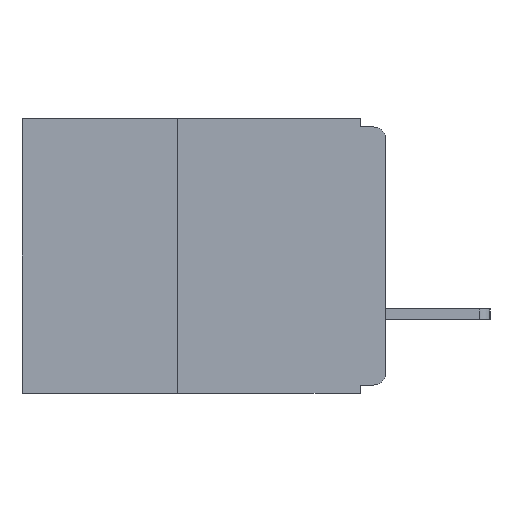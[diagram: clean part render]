
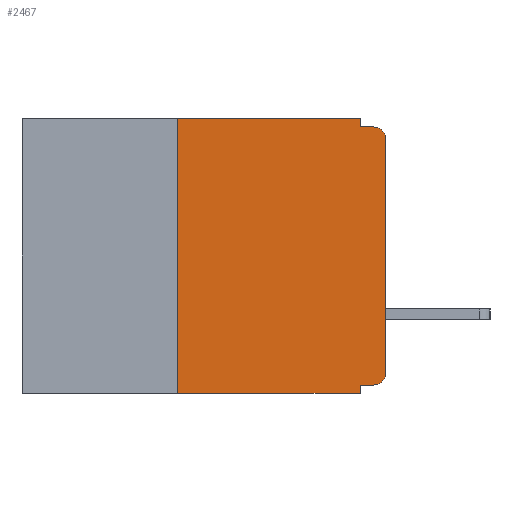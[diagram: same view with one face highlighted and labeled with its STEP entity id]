
A CAD part, left-side view. The second image highlights one B-rep face of the part: STEP entity #2467.
In plain terms, the highlighted planar face has unit normal (-1, 0, 0).
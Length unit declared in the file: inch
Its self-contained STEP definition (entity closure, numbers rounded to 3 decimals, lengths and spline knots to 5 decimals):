
#266 = DIRECTION ( 'NONE',  ( 0., 0., 1. ) ) ;
#405 = DIRECTION ( 'NONE',  ( 0., 0., -1. ) ) ;
#1133 = DIRECTION ( 'NONE',  ( -1., 0., 0. ) ) ;
#1836 = EDGE_CURVE ( 'NONE', #6928, #7403, #9628, .T. ) ;
#2467 = ADVANCED_FACE ( 'NONE', ( #5441 ), #2619, .F. ) ;
#2619 = PLANE ( 'NONE',  #10414 ) ;
#2712 = EDGE_CURVE ( 'NONE', #7403, #15019, #13500, .T. ) ;
#2730 = VECTOR ( 'NONE', #266, 39.37008 ) ;
#2902 = DIRECTION ( 'NONE',  ( 0., -1., 0. ) ) ;
#2996 = CARTESIAN_POINT ( 'NONE',  ( 0., 0.031, -0.01 ) ) ;
#3098 = EDGE_CURVE ( 'NONE', #8021, #14418, #10614, .T. ) ;
#3619 = ORIENTED_EDGE ( 'NONE', *, *, #6432, .F. ) ;
#3790 = DIRECTION ( 'NONE',  ( 0., -1., 0. ) ) ;
#4138 = CARTESIAN_POINT ( 'NONE',  ( 0., 0.015, -0.01 ) ) ;
#4578 = CARTESIAN_POINT ( 'NONE',  ( 0., 0., -0.01 ) ) ;
#4622 = VERTEX_POINT ( 'NONE', #8801 ) ;
#5047 = CARTESIAN_POINT ( 'NONE',  ( 0., 0., -0.305 ) ) ;
#5087 = VERTEX_POINT ( 'NONE', #5047 ) ;
#5209 = VECTOR ( 'NONE', #11795, 39.37008 ) ;
#5441 = FACE_OUTER_BOUND ( 'NONE', #16804, .T. ) ;
#5730 = AXIS2_PLACEMENT_3D ( 'NONE', #20215, #10373, #405 ) ;
#5821 = DIRECTION ( 'NONE',  ( 0., 0., -1. ) ) ;
#5935 = CARTESIAN_POINT ( 'NONE',  ( 0., 0., -0.32 ) ) ;
#6432 = EDGE_CURVE ( 'NONE', #18299, #6928, #12663, .T. ) ;
#6604 = ORIENTED_EDGE ( 'NONE', *, *, #2712, .F. ) ;
#6928 = VERTEX_POINT ( 'NONE', #10141 ) ;
#7403 = VERTEX_POINT ( 'NONE', #19286 ) ;
#7618 = DIRECTION ( 'NONE',  ( 0., 1., 0. ) ) ;
#8021 = VERTEX_POINT ( 'NONE', #16080 ) ;
#8182 = LINE ( 'NONE', #4578, #20773 ) ;
#8572 = CARTESIAN_POINT ( 'NONE',  ( 0., 0.25, -0.33 ) ) ;
#8801 = CARTESIAN_POINT ( 'NONE',  ( 0., 0., -0.025 ) ) ;
#9303 = DIRECTION ( 'NONE',  ( 0., 0., -1. ) ) ;
#9563 = LINE ( 'NONE', #12124, #17318 ) ;
#9628 = LINE ( 'NONE', #18093, #5209 ) ;
#9695 = ORIENTED_EDGE ( 'NONE', *, *, #14667, .T. ) ;
#9861 = CARTESIAN_POINT ( 'NONE',  ( 0., 0.031, -0.33 ) ) ;
#10141 = CARTESIAN_POINT ( 'NONE',  ( 0., 0.25, 0. ) ) ;
#10373 = DIRECTION ( 'NONE',  ( -1., 0., 0. ) ) ;
#10414 = AXIS2_PLACEMENT_3D ( 'NONE', #13671, #13317, #13174 ) ;
#10606 = CIRCLE ( 'NONE', #5730, 0.015 ) ;
#10614 = LINE ( 'NONE', #11590, #18835 ) ;
#11120 = CARTESIAN_POINT ( 'NONE',  ( 0., 0.015, -0.305 ) ) ;
#11217 = EDGE_CURVE ( 'NONE', #15019, #20081, #8182, .T. ) ;
#11358 = VECTOR ( 'NONE', #7618, 39.37008 ) ;
#11457 = CARTESIAN_POINT ( 'NONE',  ( 0., 0.031, 0. ) ) ;
#11590 = CARTESIAN_POINT ( 'NONE',  ( 0., 0.031, -0.33 ) ) ;
#11795 = DIRECTION ( 'NONE',  ( 0., -1., 0. ) ) ;
#12124 = CARTESIAN_POINT ( 'NONE',  ( 0., 0.437, -0.33 ) ) ;
#12565 = CARTESIAN_POINT ( 'NONE',  ( 0., 0.25, -0.33 ) ) ;
#12663 = LINE ( 'NONE', #8572, #2730 ) ;
#12796 = DIRECTION ( 'NONE',  ( 0., 0., -1. ) ) ;
#12972 = CIRCLE ( 'NONE', #19817, 0.015 ) ;
#13174 = DIRECTION ( 'NONE',  ( 0., 0., -1. ) ) ;
#13317 = DIRECTION ( 'NONE',  ( 1., 0., 0. ) ) ;
#13500 = LINE ( 'NONE', #11457, #18344 ) ;
#13671 = CARTESIAN_POINT ( 'NONE',  ( 0., 0.437, 0. ) ) ;
#14001 = ORIENTED_EDGE ( 'NONE', *, *, #1836, .F. ) ;
#14253 = EDGE_CURVE ( 'NONE', #19548, #5087, #12972, .T. ) ;
#14418 = VERTEX_POINT ( 'NONE', #9861 ) ;
#14619 = ORIENTED_EDGE ( 'NONE', *, *, #3098, .F. ) ;
#14622 = EDGE_CURVE ( 'NONE', #4622, #20081, #10606, .T. ) ;
#14667 = EDGE_CURVE ( 'NONE', #18299, #14418, #9563, .T. ) ;
#14772 = ORIENTED_EDGE ( 'NONE', *, *, #14622, .T. ) ;
#15019 = VERTEX_POINT ( 'NONE', #2996 ) ;
#15590 = ORIENTED_EDGE ( 'NONE', *, *, #20904, .T. ) ;
#15748 = LINE ( 'NONE', #5935, #11358 ) ;
#15926 = LINE ( 'NONE', #19869, #21267 ) ;
#15975 = CARTESIAN_POINT ( 'NONE',  ( 0., 0.015, -0.32 ) ) ;
#16080 = CARTESIAN_POINT ( 'NONE',  ( 0., 0.031, -0.32 ) ) ;
#16541 = DIRECTION ( 'NONE',  ( 0., 0., 1. ) ) ;
#16804 = EDGE_LOOP ( 'NONE', ( #15590, #14772, #19551, #6604, #14001, #3619, #9695, #14619, #20695, #20275 ) ) ;
#17318 = VECTOR ( 'NONE', #3790, 39.37008 ) ;
#18093 = CARTESIAN_POINT ( 'NONE',  ( 0., 0.437, 0. ) ) ;
#18299 = VERTEX_POINT ( 'NONE', #12565 ) ;
#18344 = VECTOR ( 'NONE', #9303, 39.37008 ) ;
#18835 = VECTOR ( 'NONE', #5821, 39.37008 ) ;
#18860 = EDGE_CURVE ( 'NONE', #19548, #8021, #15748, .T. ) ;
#19286 = CARTESIAN_POINT ( 'NONE',  ( 0., 0.031, 0. ) ) ;
#19548 = VERTEX_POINT ( 'NONE', #15975 ) ;
#19551 = ORIENTED_EDGE ( 'NONE', *, *, #11217, .F. ) ;
#19817 = AXIS2_PLACEMENT_3D ( 'NONE', #11120, #1133, #12796 ) ;
#19869 = CARTESIAN_POINT ( 'NONE',  ( 0., 0., 0. ) ) ;
#20081 = VERTEX_POINT ( 'NONE', #4138 ) ;
#20215 = CARTESIAN_POINT ( 'NONE',  ( 0., 0.015, -0.025 ) ) ;
#20275 = ORIENTED_EDGE ( 'NONE', *, *, #14253, .T. ) ;
#20695 = ORIENTED_EDGE ( 'NONE', *, *, #18860, .F. ) ;
#20773 = VECTOR ( 'NONE', #2902, 39.37008 ) ;
#20904 = EDGE_CURVE ( 'NONE', #5087, #4622, #15926, .T. ) ;
#21267 = VECTOR ( 'NONE', #16541, 39.37008 ) ;
